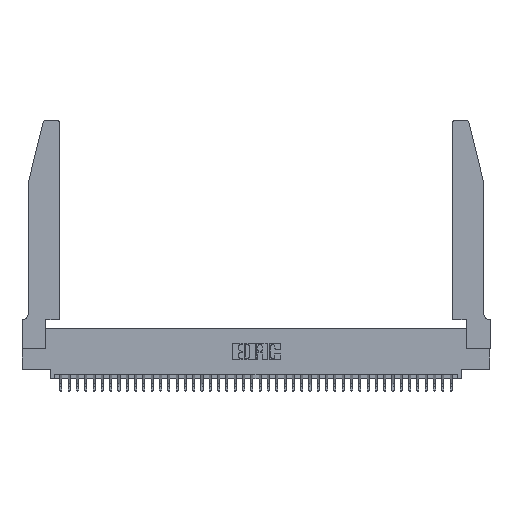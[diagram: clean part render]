
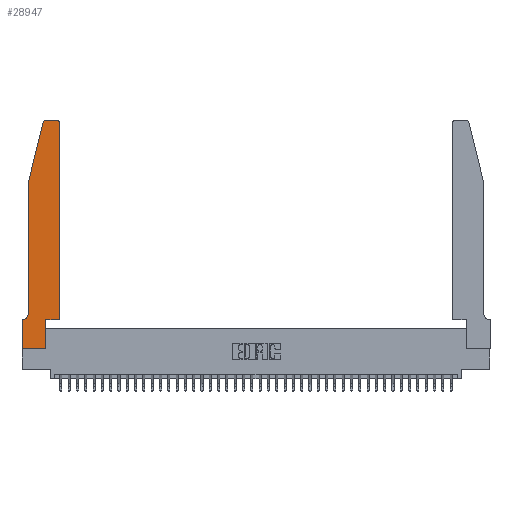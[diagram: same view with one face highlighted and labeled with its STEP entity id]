
A CAD part, top view. The second image highlights one B-rep face of the part: STEP entity #28947.
In plain terms, the highlighted planar face has unit normal (0, 0, 1).
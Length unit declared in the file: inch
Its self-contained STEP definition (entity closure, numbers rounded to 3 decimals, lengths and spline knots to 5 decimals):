
#735 = DIRECTION ( 'NONE',  ( 0., 0., 1. ) ) ;
#833 = LINE ( 'NONE', #14763, #34324 ) ;
#893 = CARTESIAN_POINT ( 'NONE',  ( 0.2865, 0., 0.37 ) ) ;
#1046 = CARTESIAN_POINT ( 'NONE',  ( 0.0055, 0.42, 0.37 ) ) ;
#1301 = VECTOR ( 'NONE', #40547, 39.37008 ) ;
#1782 = EDGE_LOOP ( 'NONE', ( #5882, #38364, #39424, #12832, #18339, #6499, #12018, #12841, #22091, #29835, #9033, #35143 ) ) ;
#2125 = VERTEX_POINT ( 'NONE', #16101 ) ;
#2512 = DIRECTION ( 'NONE',  ( 1., 0., 0. ) ) ;
#2892 = CARTESIAN_POINT ( 'NONE',  ( 0.0755, 2., 0.37 ) ) ;
#3045 = DIRECTION ( 'NONE',  ( -1., 0., 0. ) ) ;
#3803 = VECTOR ( 'NONE', #3045, 39.37008 ) ;
#4761 = AXIS2_PLACEMENT_3D ( 'NONE', #1046, #10858, #36704 ) ;
#4811 = CARTESIAN_POINT ( 'NONE',  ( 0.4505, 0.35, 0.37 ) ) ;
#5568 = CARTESIAN_POINT ( 'NONE',  ( 0.4505, 0.35, 0.37 ) ) ;
#5650 = CARTESIAN_POINT ( 'NONE',  ( 0., 0.35, 0.37 ) ) ;
#5882 = ORIENTED_EDGE ( 'NONE', *, *, #35247, .T. ) ;
#6499 = ORIENTED_EDGE ( 'NONE', *, *, #20711, .T. ) ;
#7120 = EDGE_CURVE ( 'NONE', #15540, #10046, #29082, .T. ) ;
#7394 = LINE ( 'NONE', #5568, #7883 ) ;
#7883 = VECTOR ( 'NONE', #41005, 39.37008 ) ;
#8443 = LINE ( 'NONE', #31087, #1301 ) ;
#9033 = ORIENTED_EDGE ( 'NONE', *, *, #20426, .T. ) ;
#9352 = VECTOR ( 'NONE', #41007, 39.37008 ) ;
#9561 = EDGE_CURVE ( 'NONE', #28836, #36509, #12392, .T. ) ;
#9746 = DIRECTION ( 'NONE',  ( 1., 0., 0. ) ) ;
#9822 = LINE ( 'NONE', #18564, #9352 ) ;
#10046 = VERTEX_POINT ( 'NONE', #14423 ) ;
#10708 = VERTEX_POINT ( 'NONE', #4811 ) ;
#10832 = EDGE_CURVE ( 'NONE', #13722, #19502, #14743, .T. ) ;
#10858 = DIRECTION ( 'NONE',  ( 0., 0., -1. ) ) ;
#12015 = CARTESIAN_POINT ( 'NONE',  ( 0.284, 2.72, 0.37 ) ) ;
#12018 = ORIENTED_EDGE ( 'NONE', *, *, #9561, .T. ) ;
#12392 = LINE ( 'NONE', #29018, #41774 ) ;
#12832 = ORIENTED_EDGE ( 'NONE', *, *, #7120, .T. ) ;
#12841 = ORIENTED_EDGE ( 'NONE', *, *, #28304, .T. ) ;
#13054 = DIRECTION ( 'NONE',  ( 1., 0., 0. ) ) ;
#13722 = VERTEX_POINT ( 'NONE', #19389 ) ;
#14149 = CARTESIAN_POINT ( 'NONE',  ( 0.2605, 2.75, 0.37 ) ) ;
#14423 = CARTESIAN_POINT ( 'NONE',  ( 0.0755, 0.42, 0.37 ) ) ;
#14743 = CIRCLE ( 'NONE', #32264, 0.03 ) ;
#14763 = CARTESIAN_POINT ( 'NONE',  ( 0.0755, 2., 0.37 ) ) ;
#14901 = CARTESIAN_POINT ( 'NONE',  ( 0.4205, 2.75, 0.37 ) ) ;
#15215 = AXIS2_PLACEMENT_3D ( 'NONE', #5650, #28278, #9746 ) ;
#15231 = PLANE ( 'NONE',  #15215 ) ;
#15540 = VERTEX_POINT ( 'NONE', #2892 ) ;
#16101 = CARTESIAN_POINT ( 'NONE',  ( 0.0055, 0.35, 0.37 ) ) ;
#16114 = CARTESIAN_POINT ( 'NONE',  ( 0., 0., 0.37 ) ) ;
#16885 = FACE_OUTER_BOUND ( 'NONE', #1782, .T. ) ;
#17276 = CIRCLE ( 'NONE', #4761, 0.07 ) ;
#17502 = EDGE_CURVE ( 'NONE', #40639, #37292, #36984, .T. ) ;
#18339 = ORIENTED_EDGE ( 'NONE', *, *, #22335, .T. ) ;
#18564 = CARTESIAN_POINT ( 'NONE',  ( 0.2865, 0.35, 0.37 ) ) ;
#18611 = DIRECTION ( 'NONE',  ( 1., 0., 0. ) ) ;
#19389 = CARTESIAN_POINT ( 'NONE',  ( 0.4505, 2.72, 0.37 ) ) ;
#19472 = EDGE_CURVE ( 'NONE', #37292, #15540, #833, .T. ) ;
#19502 = VERTEX_POINT ( 'NONE', #14901 ) ;
#20426 = EDGE_CURVE ( 'NONE', #10708, #13722, #8443, .T. ) ;
#20711 = EDGE_CURVE ( 'NONE', #2125, #28836, #33196, .T. ) ;
#21843 = CARTESIAN_POINT ( 'NONE',  ( 0.0755, 0.35, 0.37 ) ) ;
#22091 = ORIENTED_EDGE ( 'NONE', *, *, #34849, .T. ) ;
#22335 = EDGE_CURVE ( 'NONE', #10046, #2125, #17276, .T. ) ;
#22347 = DIRECTION ( 'NONE',  ( 0., -1., 0. ) ) ;
#22425 = CARTESIAN_POINT ( 'NONE',  ( 0.4205, 2.72, 0.37 ) ) ;
#23082 = AXIS2_PLACEMENT_3D ( 'NONE', #12015, #34659, #2512 ) ;
#24971 = DIRECTION ( 'NONE',  ( -0.239, -0.971, 0. ) ) ;
#25584 = CARTESIAN_POINT ( 'NONE',  ( 0., 0.35, 0.37 ) ) ;
#26019 = VECTOR ( 'NONE', #27028, 39.37008 ) ;
#27028 = DIRECTION ( 'NONE',  ( 0., -1., 0. ) ) ;
#27922 = CARTESIAN_POINT ( 'NONE',  ( 0.25487, 2.72718, 0.37 ) ) ;
#28122 = EDGE_CURVE ( 'NONE', #31008, #10708, #7394, .T. ) ;
#28278 = DIRECTION ( 'NONE',  ( 0., 0., 1. ) ) ;
#28304 = EDGE_CURVE ( 'NONE', #36509, #31406, #40879, .T. ) ;
#28836 = VERTEX_POINT ( 'NONE', #25584 ) ;
#28947 = ADVANCED_FACE ( 'NONE', ( #16885 ), #15231, .T. ) ;
#29018 = CARTESIAN_POINT ( 'NONE',  ( 0., 0., 0.37 ) ) ;
#29082 = LINE ( 'NONE', #37098, #26019 ) ;
#29835 = ORIENTED_EDGE ( 'NONE', *, *, #28122, .T. ) ;
#31001 = CARTESIAN_POINT ( 'NONE',  ( 0.284, 2.75, 0.37 ) ) ;
#31008 = VERTEX_POINT ( 'NONE', #39180 ) ;
#31087 = CARTESIAN_POINT ( 'NONE',  ( 0.4505, 0.35, 0.37 ) ) ;
#31406 = VERTEX_POINT ( 'NONE', #893 ) ;
#32264 = AXIS2_PLACEMENT_3D ( 'NONE', #22425, #735, #18611 ) ;
#33196 = LINE ( 'NONE', #21843, #3803 ) ;
#34324 = VECTOR ( 'NONE', #24971, 39.37008 ) ;
#34659 = DIRECTION ( 'NONE',  ( 0., 0., 1. ) ) ;
#34849 = EDGE_CURVE ( 'NONE', #31406, #31008, #9822, .T. ) ;
#35122 = VECTOR ( 'NONE', #36769, 39.37008 ) ;
#35143 = ORIENTED_EDGE ( 'NONE', *, *, #10832, .T. ) ;
#35247 = EDGE_CURVE ( 'NONE', #19502, #40639, #37135, .T. ) ;
#36509 = VERTEX_POINT ( 'NONE', #37499 ) ;
#36704 = DIRECTION ( 'NONE',  ( -1., 0., 0. ) ) ;
#36769 = DIRECTION ( 'NONE',  ( -1., 0., 0. ) ) ;
#36984 = CIRCLE ( 'NONE', #23082, 0.03 ) ;
#37098 = CARTESIAN_POINT ( 'NONE',  ( 0.0755, 2., 0.37 ) ) ;
#37135 = LINE ( 'NONE', #14149, #35122 ) ;
#37292 = VERTEX_POINT ( 'NONE', #27922 ) ;
#37499 = CARTESIAN_POINT ( 'NONE',  ( 0., 0., 0.37 ) ) ;
#38364 = ORIENTED_EDGE ( 'NONE', *, *, #17502, .T. ) ;
#39180 = CARTESIAN_POINT ( 'NONE',  ( 0.2865, 0.35, 0.37 ) ) ;
#39424 = ORIENTED_EDGE ( 'NONE', *, *, #19472, .T. ) ;
#40547 = DIRECTION ( 'NONE',  ( 0., 1., 0. ) ) ;
#40639 = VERTEX_POINT ( 'NONE', #31001 ) ;
#40879 = LINE ( 'NONE', #16114, #41862 ) ;
#41005 = DIRECTION ( 'NONE',  ( 1., 0., 0. ) ) ;
#41007 = DIRECTION ( 'NONE',  ( 0., 1., 0. ) ) ;
#41774 = VECTOR ( 'NONE', #22347, 39.37008 ) ;
#41862 = VECTOR ( 'NONE', #13054, 39.37008 ) ;
